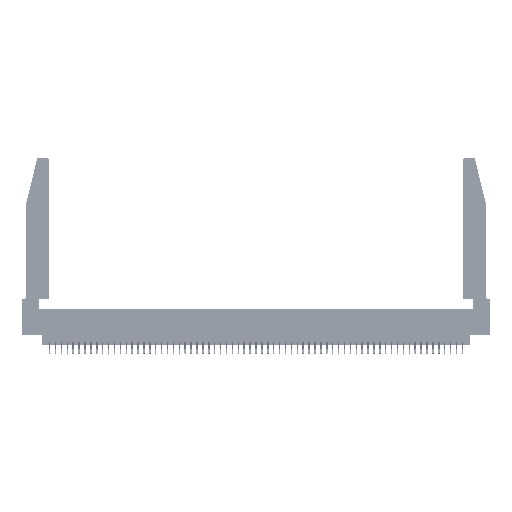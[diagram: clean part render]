
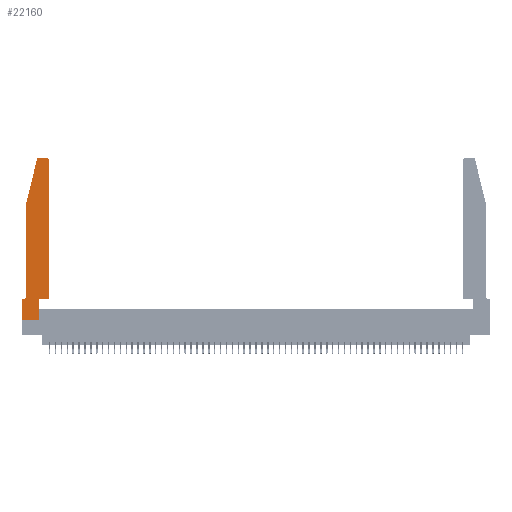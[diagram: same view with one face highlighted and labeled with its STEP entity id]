
A CAD part, top view. The second image highlights one B-rep face of the part: STEP entity #22160.
In plain terms, the highlighted planar face has unit normal (0, 0, 1).
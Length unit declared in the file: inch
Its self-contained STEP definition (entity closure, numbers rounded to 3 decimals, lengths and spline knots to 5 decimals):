
#799 = ORIENTED_EDGE ( 'NONE', *, *, #20446, .T. ) ;
#818 = EDGE_CURVE ( 'NONE', #12034, #31268, #51766, .T. ) ;
#1296 = FACE_OUTER_BOUND ( 'NONE', #7865, .T. ) ;
#1767 = CARTESIAN_POINT ( 'NONE',  ( 0.0055, 0.35, 0.37 ) ) ;
#2480 = CARTESIAN_POINT ( 'NONE',  ( 0., 0.35, 0.37 ) ) ;
#2507 = VERTEX_POINT ( 'NONE', #2480 ) ;
#2732 = EDGE_CURVE ( 'NONE', #26675, #43189, #18137, .T. ) ;
#3456 = CARTESIAN_POINT ( 'NONE',  ( 0.4205, 2.75, 0.37 ) ) ;
#5259 = CARTESIAN_POINT ( 'NONE',  ( 0.0755, 2., 0.37 ) ) ;
#6942 = CARTESIAN_POINT ( 'NONE',  ( 0.2865, 0., 0.37 ) ) ;
#7602 = DIRECTION ( 'NONE',  ( 1., 0., 0. ) ) ;
#7865 = EDGE_LOOP ( 'NONE', ( #39095, #16059, #17488, #51557, #27128, #799, #9885, #43691, #22592, #31531, #13663, #23429 ) ) ;
#7883 = EDGE_CURVE ( 'NONE', #2507, #26675, #26254, .T. ) ;
#8384 = EDGE_CURVE ( 'NONE', #31268, #44921, #49235, .T. ) ;
#8602 = CARTESIAN_POINT ( 'NONE',  ( 0.4505, 0.35, 0.37 ) ) ;
#8650 = CARTESIAN_POINT ( 'NONE',  ( 0.25487, 2.72718, 0.37 ) ) ;
#9885 = ORIENTED_EDGE ( 'NONE', *, *, #7883, .T. ) ;
#10943 = LINE ( 'NONE', #15570, #43176 ) ;
#11570 = CARTESIAN_POINT ( 'NONE',  ( 0., 0., 0.37 ) ) ;
#12034 = VERTEX_POINT ( 'NONE', #15001 ) ;
#13184 = DIRECTION ( 'NONE',  ( 1., 0., 0. ) ) ;
#13285 = CARTESIAN_POINT ( 'NONE',  ( 0., 0.35, 0.37 ) ) ;
#13663 = ORIENTED_EDGE ( 'NONE', *, *, #17834, .T. ) ;
#14557 = CARTESIAN_POINT ( 'NONE',  ( 0.4205, 2.72, 0.37 ) ) ;
#15001 = CARTESIAN_POINT ( 'NONE',  ( 0.0755, 2., 0.37 ) ) ;
#15570 = CARTESIAN_POINT ( 'NONE',  ( 0.2865, 0.35, 0.37 ) ) ;
#15905 = CARTESIAN_POINT ( 'NONE',  ( 0.284, 2.72, 0.37 ) ) ;
#16059 = ORIENTED_EDGE ( 'NONE', *, *, #26065, .T. ) ;
#16281 = CARTESIAN_POINT ( 'NONE',  ( 0., 0., 0.37 ) ) ;
#16626 = DIRECTION ( 'NONE',  ( -0.239, -0.971, 0. ) ) ;
#17018 = VECTOR ( 'NONE', #40532, 39.37008 ) ;
#17488 = ORIENTED_EDGE ( 'NONE', *, *, #49453, .T. ) ;
#17834 = EDGE_CURVE ( 'NONE', #40090, #43894, #30933, .T. ) ;
#18137 = LINE ( 'NONE', #39413, #20900 ) ;
#18856 = CIRCLE ( 'NONE', #34405, 0.03 ) ;
#19026 = DIRECTION ( 'NONE',  ( 1., 0., 0. ) ) ;
#19134 = VERTEX_POINT ( 'NONE', #3456 ) ;
#19804 = LINE ( 'NONE', #34887, #21202 ) ;
#20365 = DIRECTION ( 'NONE',  ( 1., 0., 0. ) ) ;
#20446 = EDGE_CURVE ( 'NONE', #44921, #2507, #19804, .T. ) ;
#20615 = CIRCLE ( 'NONE', #26091, 0.03 ) ;
#20756 = DIRECTION ( 'NONE',  ( 0., -1., 0. ) ) ;
#20900 = VECTOR ( 'NONE', #13184, 39.37008 ) ;
#21104 = VERTEX_POINT ( 'NONE', #8650 ) ;
#21202 = VECTOR ( 'NONE', #52178, 39.37008 ) ;
#22160 = ADVANCED_FACE ( 'NONE', ( #1296 ), #48164, .T. ) ;
#22592 = ORIENTED_EDGE ( 'NONE', *, *, #25381, .T. ) ;
#23429 = ORIENTED_EDGE ( 'NONE', *, *, #47265, .T. ) ;
#23591 = VERTEX_POINT ( 'NONE', #45356 ) ;
#24263 = DIRECTION ( 'NONE',  ( 0., 1., 0. ) ) ;
#24535 = CARTESIAN_POINT ( 'NONE',  ( 0.0055, 0.42, 0.37 ) ) ;
#25381 = EDGE_CURVE ( 'NONE', #43189, #23591, #10943, .T. ) ;
#26065 = EDGE_CURVE ( 'NONE', #31977, #21104, #20615, .T. ) ;
#26091 = AXIS2_PLACEMENT_3D ( 'NONE', #15905, #46372, #20365 ) ;
#26254 = LINE ( 'NONE', #16281, #47950 ) ;
#26551 = DIRECTION ( 'NONE',  ( 1., 0., 0. ) ) ;
#26675 = VERTEX_POINT ( 'NONE', #11570 ) ;
#27128 = ORIENTED_EDGE ( 'NONE', *, *, #8384, .T. ) ;
#28618 = LINE ( 'NONE', #46883, #38851 ) ;
#28892 = DIRECTION ( 'NONE',  ( -1., 0., 0. ) ) ;
#29641 = CARTESIAN_POINT ( 'NONE',  ( 0.4505, 0.35, 0.37 ) ) ;
#30933 = LINE ( 'NONE', #33777, #41123 ) ;
#31268 = VERTEX_POINT ( 'NONE', #49755 ) ;
#31531 = ORIENTED_EDGE ( 'NONE', *, *, #49436, .T. ) ;
#31561 = VECTOR ( 'NONE', #16626, 39.37008 ) ;
#31977 = VERTEX_POINT ( 'NONE', #54247 ) ;
#33777 = CARTESIAN_POINT ( 'NONE',  ( 0.4505, 0.35, 0.37 ) ) ;
#34018 = CARTESIAN_POINT ( 'NONE',  ( 0.0755, 2., 0.37 ) ) ;
#34405 = AXIS2_PLACEMENT_3D ( 'NONE', #14557, #45061, #19026 ) ;
#34887 = CARTESIAN_POINT ( 'NONE',  ( 0.0755, 0.35, 0.37 ) ) ;
#37244 = AXIS2_PLACEMENT_3D ( 'NONE', #13285, #52587, #26551 ) ;
#38180 = DIRECTION ( 'NONE',  ( 0., 1., 0. ) ) ;
#38851 = VECTOR ( 'NONE', #51098, 39.37008 ) ;
#39095 = ORIENTED_EDGE ( 'NONE', *, *, #51365, .T. ) ;
#39413 = CARTESIAN_POINT ( 'NONE',  ( 0., 0., 0.37 ) ) ;
#40090 = VERTEX_POINT ( 'NONE', #8602 ) ;
#40532 = DIRECTION ( 'NONE',  ( 0., -1., 0. ) ) ;
#41123 = VECTOR ( 'NONE', #38180, 39.37008 ) ;
#43128 = LINE ( 'NONE', #34018, #31561 ) ;
#43176 = VECTOR ( 'NONE', #24263, 39.37008 ) ;
#43189 = VERTEX_POINT ( 'NONE', #6942 ) ;
#43691 = ORIENTED_EDGE ( 'NONE', *, *, #2732, .T. ) ;
#43894 = VERTEX_POINT ( 'NONE', #51138 ) ;
#44457 = LINE ( 'NONE', #29641, #45782 ) ;
#44921 = VERTEX_POINT ( 'NONE', #1767 ) ;
#45061 = DIRECTION ( 'NONE',  ( 0., 0., 1. ) ) ;
#45356 = CARTESIAN_POINT ( 'NONE',  ( 0.2865, 0.35, 0.37 ) ) ;
#45782 = VECTOR ( 'NONE', #7602, 39.37008 ) ;
#46372 = DIRECTION ( 'NONE',  ( 0., 0., 1. ) ) ;
#46883 = CARTESIAN_POINT ( 'NONE',  ( 0.2605, 2.75, 0.37 ) ) ;
#47265 = EDGE_CURVE ( 'NONE', #43894, #19134, #18856, .T. ) ;
#47950 = VECTOR ( 'NONE', #20756, 39.37008 ) ;
#48164 = PLANE ( 'NONE',  #37244 ) ;
#49235 = CIRCLE ( 'NONE', #53192, 0.07 ) ;
#49436 = EDGE_CURVE ( 'NONE', #23591, #40090, #44457, .T. ) ;
#49453 = EDGE_CURVE ( 'NONE', #21104, #12034, #43128, .T. ) ;
#49755 = CARTESIAN_POINT ( 'NONE',  ( 0.0755, 0.42, 0.37 ) ) ;
#51098 = DIRECTION ( 'NONE',  ( -1., 0., 0. ) ) ;
#51138 = CARTESIAN_POINT ( 'NONE',  ( 0.4505, 2.72, 0.37 ) ) ;
#51365 = EDGE_CURVE ( 'NONE', #19134, #31977, #28618, .T. ) ;
#51557 = ORIENTED_EDGE ( 'NONE', *, *, #818, .T. ) ;
#51766 = LINE ( 'NONE', #5259, #17018 ) ;
#52178 = DIRECTION ( 'NONE',  ( -1., 0., 0. ) ) ;
#52587 = DIRECTION ( 'NONE',  ( 0., 0., 1. ) ) ;
#53192 = AXIS2_PLACEMENT_3D ( 'NONE', #24535, #54867, #28892 ) ;
#54247 = CARTESIAN_POINT ( 'NONE',  ( 0.284, 2.75, 0.37 ) ) ;
#54867 = DIRECTION ( 'NONE',  ( 0., 0., -1. ) ) ;
